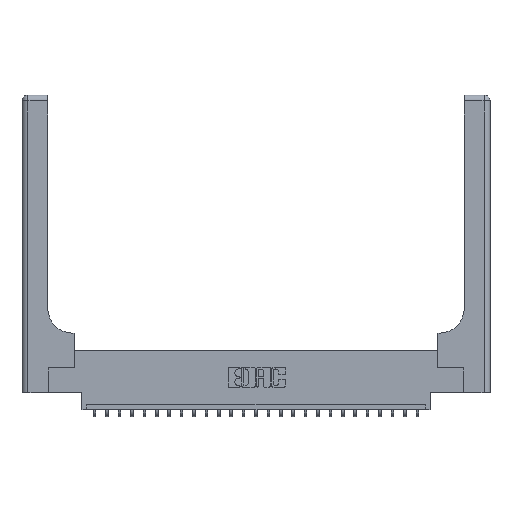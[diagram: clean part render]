
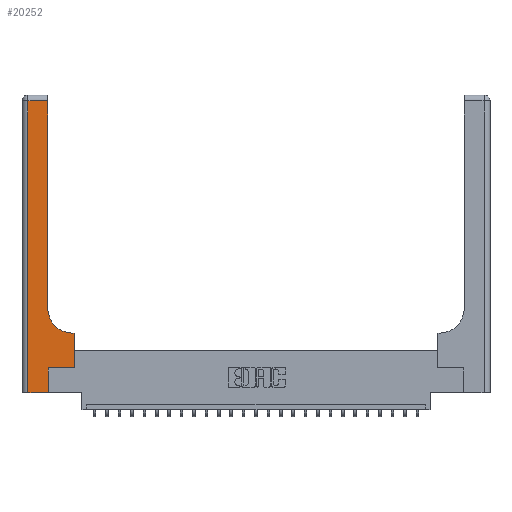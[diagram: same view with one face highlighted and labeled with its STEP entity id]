
A CAD part, top view. The second image highlights one B-rep face of the part: STEP entity #20252.
In plain terms, the highlighted planar face has unit normal (0, 0, 1).
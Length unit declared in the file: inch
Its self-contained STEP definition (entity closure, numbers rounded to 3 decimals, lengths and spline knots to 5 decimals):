
#55 = CIRCLE ( 'NONE', #13261, 0.25 ) ;
#901 = EDGE_CURVE ( 'NONE', #19037, #3834, #21793, .T. ) ;
#1007 = EDGE_CURVE ( 'NONE', #1946, #5923, #20038, .T. ) ;
#1423 = VERTEX_POINT ( 'NONE', #21668 ) ;
#1946 = VERTEX_POINT ( 'NONE', #3589 ) ;
#2030 = VERTEX_POINT ( 'NONE', #18764 ) ;
#3060 = CARTESIAN_POINT ( 'NONE',  ( 0., 0., 0.37 ) ) ;
#3589 = CARTESIAN_POINT ( 'NONE',  ( 0.06, 2.94, 0.37 ) ) ;
#3834 = VERTEX_POINT ( 'NONE', #11296 ) ;
#4695 = LINE ( 'NONE', #5367, #23287 ) ;
#5154 = VECTOR ( 'NONE', #15033, 39.37008 ) ;
#5347 = DIRECTION ( 'NONE',  ( 0., -1., 0. ) ) ;
#5367 = CARTESIAN_POINT ( 'NONE',  ( 0., 2.94, 0.37 ) ) ;
#5715 = CARTESIAN_POINT ( 'NONE',  ( 0.26, 2.94, 0.37 ) ) ;
#5923 = VERTEX_POINT ( 'NONE', #20284 ) ;
#6487 = FACE_OUTER_BOUND ( 'NONE', #18220, .T. ) ;
#6996 = VECTOR ( 'NONE', #21829, 39.37008 ) ;
#7211 = ORIENTED_EDGE ( 'NONE', *, *, #1007, .T. ) ;
#7271 = DIRECTION ( 'NONE',  ( -1., 0., 0. ) ) ;
#7386 = DIRECTION ( 'NONE',  ( 0., 0., -1. ) ) ;
#8338 = CARTESIAN_POINT ( 'NONE',  ( 0.265, 0.25, 0.37 ) ) ;
#8655 = EDGE_CURVE ( 'NONE', #9064, #1423, #55, .T. ) ;
#9017 = ORIENTED_EDGE ( 'NONE', *, *, #19560, .T. ) ;
#9064 = VERTEX_POINT ( 'NONE', #19620 ) ;
#9178 = CARTESIAN_POINT ( 'NONE',  ( 0.06, 3., 0.37 ) ) ;
#9633 = CARTESIAN_POINT ( 'NONE',  ( 0., 3., 0.37 ) ) ;
#10230 = ORIENTED_EDGE ( 'NONE', *, *, #8655, .T. ) ;
#10296 = VECTOR ( 'NONE', #5347, 39.37008 ) ;
#10841 = DIRECTION ( 'NONE',  ( -1., 0., 0. ) ) ;
#11296 = CARTESIAN_POINT ( 'NONE',  ( 0.528, 0.25, 0.37 ) ) ;
#11515 = DIRECTION ( 'NONE',  ( -1., 0., 0. ) ) ;
#11652 = ORIENTED_EDGE ( 'NONE', *, *, #21981, .T. ) ;
#11690 = CARTESIAN_POINT ( 'NONE',  ( 0.528, 0.25, 0.37 ) ) ;
#11820 = LINE ( 'NONE', #11690, #20425 ) ;
#12676 = CARTESIAN_POINT ( 'NONE',  ( 0.265, 0.25, 0.37 ) ) ;
#13180 = DIRECTION ( 'NONE',  ( 0., 1., 0. ) ) ;
#13190 = CARTESIAN_POINT ( 'NONE',  ( 0.265, 0., 0.37 ) ) ;
#13261 = AXIS2_PLACEMENT_3D ( 'NONE', #18513, #7386, #20349 ) ;
#13370 = ORIENTED_EDGE ( 'NONE', *, *, #16866, .T. ) ;
#13635 = EDGE_CURVE ( 'NONE', #20128, #1946, #4695, .T. ) ;
#14283 = LINE ( 'NONE', #19138, #24073 ) ;
#14510 = ORIENTED_EDGE ( 'NONE', *, *, #19246, .T. ) ;
#15033 = DIRECTION ( 'NONE',  ( 0., 1., 0. ) ) ;
#15098 = LINE ( 'NONE', #13190, #5154 ) ;
#15305 = VECTOR ( 'NONE', #16162, 39.37008 ) ;
#16162 = DIRECTION ( 'NONE',  ( 1., 0., 0. ) ) ;
#16866 = EDGE_CURVE ( 'NONE', #2030, #19037, #15098, .T. ) ;
#17110 = AXIS2_PLACEMENT_3D ( 'NONE', #9633, #22504, #11515 ) ;
#17116 = ORIENTED_EDGE ( 'NONE', *, *, #18486, .T. ) ;
#18220 = EDGE_LOOP ( 'NONE', ( #11652, #21446, #7211, #17116, #13370, #23152, #9017, #14510, #10230 ) ) ;
#18486 = EDGE_CURVE ( 'NONE', #5923, #2030, #19050, .T. ) ;
#18513 = CARTESIAN_POINT ( 'NONE',  ( 0.51, 0.85, 0.37 ) ) ;
#18764 = CARTESIAN_POINT ( 'NONE',  ( 0.265, 0., 0.37 ) ) ;
#19037 = VERTEX_POINT ( 'NONE', #8338 ) ;
#19050 = LINE ( 'NONE', #3060, #15305 ) ;
#19138 = CARTESIAN_POINT ( 'NONE',  ( 0.26, 3., 0.37 ) ) ;
#19246 = EDGE_CURVE ( 'NONE', #21335, #9064, #23037, .T. ) ;
#19560 = EDGE_CURVE ( 'NONE', #3834, #21335, #11820, .T. ) ;
#19620 = CARTESIAN_POINT ( 'NONE',  ( 0.51, 0.6, 0.37 ) ) ;
#20038 = LINE ( 'NONE', #9178, #10296 ) ;
#20128 = VERTEX_POINT ( 'NONE', #5715 ) ;
#20252 = ADVANCED_FACE ( 'NONE', ( #6487 ), #20666, .F. ) ;
#20284 = CARTESIAN_POINT ( 'NONE',  ( 0.06, 0., 0.37 ) ) ;
#20349 = DIRECTION ( 'NONE',  ( 1., 0., 0. ) ) ;
#20425 = VECTOR ( 'NONE', #20928, 39.37008 ) ;
#20666 = PLANE ( 'NONE',  #17110 ) ;
#20928 = DIRECTION ( 'NONE',  ( 0., 1., 0. ) ) ;
#21335 = VERTEX_POINT ( 'NONE', #22206 ) ;
#21446 = ORIENTED_EDGE ( 'NONE', *, *, #13635, .T. ) ;
#21668 = CARTESIAN_POINT ( 'NONE',  ( 0.26, 0.85, 0.37 ) ) ;
#21793 = LINE ( 'NONE', #12676, #6996 ) ;
#21829 = DIRECTION ( 'NONE',  ( 1., 0., 0. ) ) ;
#21884 = VECTOR ( 'NONE', #10841, 39.37008 ) ;
#21981 = EDGE_CURVE ( 'NONE', #1423, #20128, #14283, .T. ) ;
#22206 = CARTESIAN_POINT ( 'NONE',  ( 0.528, 0.6, 0.37 ) ) ;
#22504 = DIRECTION ( 'NONE',  ( 0., 0., -1. ) ) ;
#23037 = LINE ( 'NONE', #23684, #21884 ) ;
#23152 = ORIENTED_EDGE ( 'NONE', *, *, #901, .T. ) ;
#23287 = VECTOR ( 'NONE', #7271, 39.37008 ) ;
#23684 = CARTESIAN_POINT ( 'NONE',  ( 0.26, 0.6, 0.37 ) ) ;
#24073 = VECTOR ( 'NONE', #13180, 39.37008 ) ;
